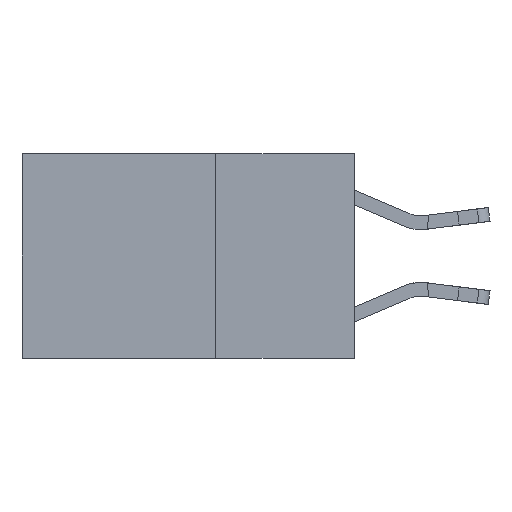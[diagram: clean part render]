
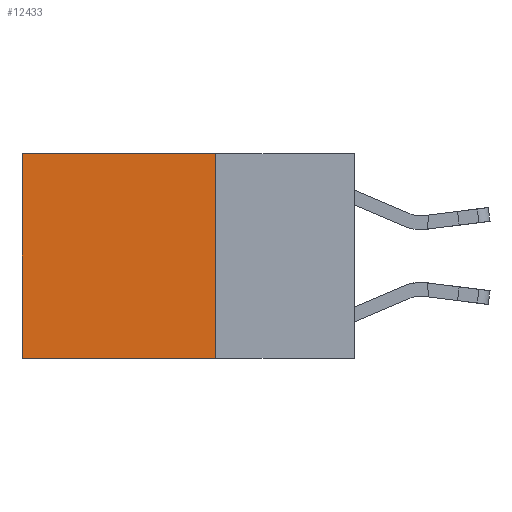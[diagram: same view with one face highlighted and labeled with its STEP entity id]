
A CAD part, left-side view. The second image highlights one B-rep face of the part: STEP entity #12433.
In plain terms, the highlighted planar face has unit normal (-1, 0, 0).
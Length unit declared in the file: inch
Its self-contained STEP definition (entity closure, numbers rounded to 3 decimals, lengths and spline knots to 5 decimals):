
#1396 = EDGE_CURVE ( 'NONE', #2272, #11136, #6994, .T. ) ;
#2272 = VERTEX_POINT ( 'NONE', #10028 ) ;
#2926 = CARTESIAN_POINT ( 'NONE',  ( 0.2625, 0.6, 0. ) ) ;
#3893 = EDGE_LOOP ( 'NONE', ( #17112, #14562, #19992, #17039 ) ) ;
#4343 = LINE ( 'NONE', #2926, #8819 ) ;
#5416 = PLANE ( 'NONE',  #6263 ) ;
#6130 = VECTOR ( 'NONE', #6784, 39.37008 ) ;
#6263 = AXIS2_PLACEMENT_3D ( 'NONE', #12066, #18676, #10412 ) ;
#6687 = DIRECTION ( 'NONE',  ( 0., 0., -1. ) ) ;
#6784 = DIRECTION ( 'NONE',  ( 0., 1., 0. ) ) ;
#6994 = LINE ( 'NONE', #15159, #6130 ) ;
#7153 = CARTESIAN_POINT ( 'NONE',  ( 0.2625, 0.6, -0.37 ) ) ;
#7386 = VERTEX_POINT ( 'NONE', #20784 ) ;
#7760 = LINE ( 'NONE', #17753, #8531 ) ;
#8531 = VECTOR ( 'NONE', #18946, 39.37008 ) ;
#8540 = CARTESIAN_POINT ( 'NONE',  ( 0.2625, 0.6, 0. ) ) ;
#8819 = VECTOR ( 'NONE', #10977, 39.37008 ) ;
#9901 = VECTOR ( 'NONE', #6687, 39.37008 ) ;
#10028 = CARTESIAN_POINT ( 'NONE',  ( 0.2625, 0.25, -0.37 ) ) ;
#10412 = DIRECTION ( 'NONE',  ( 0., 0., -1. ) ) ;
#10977 = DIRECTION ( 'NONE',  ( 0., 0., -1. ) ) ;
#11136 = VERTEX_POINT ( 'NONE', #7153 ) ;
#12066 = CARTESIAN_POINT ( 'NONE',  ( 0.2625, 0.25, 0. ) ) ;
#12433 = ADVANCED_FACE ( 'NONE', ( #16741 ), #5416, .F. ) ;
#12798 = VERTEX_POINT ( 'NONE', #8540 ) ;
#14562 = ORIENTED_EDGE ( 'NONE', *, *, #1396, .F. ) ;
#15159 = CARTESIAN_POINT ( 'NONE',  ( 0.2625, 0.25, -0.37 ) ) ;
#15404 = EDGE_CURVE ( 'NONE', #12798, #11136, #4343, .T. ) ;
#16373 = EDGE_CURVE ( 'NONE', #7386, #2272, #18315, .T. ) ;
#16616 = EDGE_CURVE ( 'NONE', #7386, #12798, #7760, .T. ) ;
#16741 = FACE_OUTER_BOUND ( 'NONE', #3893, .T. ) ;
#17039 = ORIENTED_EDGE ( 'NONE', *, *, #16616, .T. ) ;
#17112 = ORIENTED_EDGE ( 'NONE', *, *, #15404, .T. ) ;
#17753 = CARTESIAN_POINT ( 'NONE',  ( 0.2625, 0.25, 0. ) ) ;
#18315 = LINE ( 'NONE', #19526, #9901 ) ;
#18676 = DIRECTION ( 'NONE',  ( 1., 0., 0. ) ) ;
#18946 = DIRECTION ( 'NONE',  ( 0., 1., 0. ) ) ;
#19526 = CARTESIAN_POINT ( 'NONE',  ( 0.2625, 0.25, 0. ) ) ;
#19992 = ORIENTED_EDGE ( 'NONE', *, *, #16373, .F. ) ;
#20784 = CARTESIAN_POINT ( 'NONE',  ( 0.2625, 0.25, 0. ) ) ;
